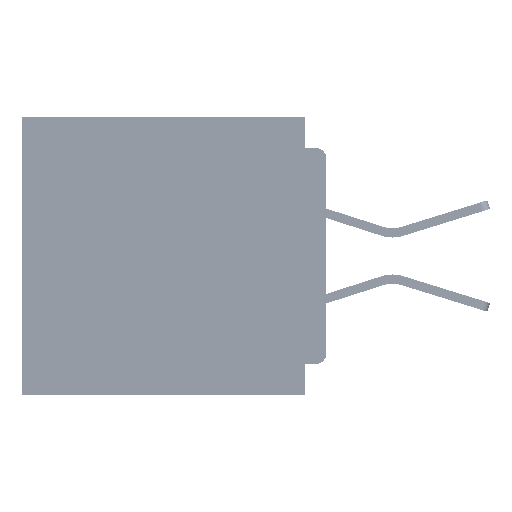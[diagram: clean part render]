
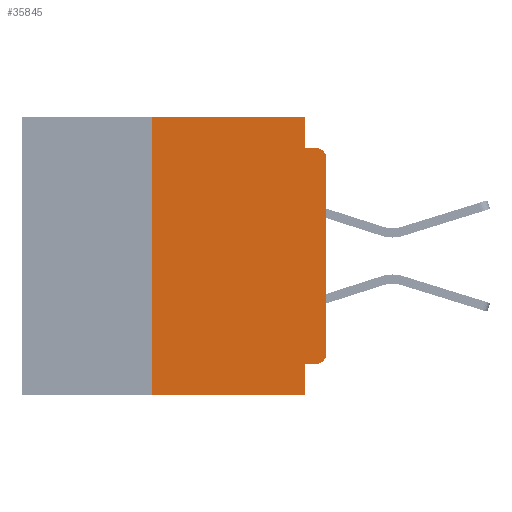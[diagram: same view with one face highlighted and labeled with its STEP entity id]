
A CAD part, left-side view. The second image highlights one B-rep face of the part: STEP entity #35845.
In plain terms, the highlighted planar face has unit normal (-1, 0, 0).
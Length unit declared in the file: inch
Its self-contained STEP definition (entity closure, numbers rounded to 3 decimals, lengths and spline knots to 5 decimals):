
#244 = CARTESIAN_POINT ( 'NONE',  ( 0., 0.015, -0.355 ) ) ;
#1551 = ORIENTED_EDGE ( 'NONE', *, *, #63702, .T. ) ;
#1789 = EDGE_CURVE ( 'NONE', #35797, #10328, #59386, .T. ) ;
#1806 = LINE ( 'NONE', #19027, #3390 ) ;
#1905 = CARTESIAN_POINT ( 'NONE',  ( 0., 0.031, 0. ) ) ;
#1924 = ORIENTED_EDGE ( 'NONE', *, *, #1789, .F. ) ;
#2128 = LINE ( 'NONE', #11401, #40152 ) ;
#2168 = CARTESIAN_POINT ( 'NONE',  ( 0., 0.015, -0.06 ) ) ;
#2187 = VECTOR ( 'NONE', #39915, 39.37008 ) ;
#2504 = CARTESIAN_POINT ( 'NONE',  ( 0., 0., -0.34 ) ) ;
#2938 = CARTESIAN_POINT ( 'NONE',  ( 0., 0.437, 0. ) ) ;
#3390 = VECTOR ( 'NONE', #53402, 39.37008 ) ;
#4965 = LINE ( 'NONE', #25827, #50999 ) ;
#5043 = VERTEX_POINT ( 'NONE', #46649 ) ;
#5642 = VERTEX_POINT ( 'NONE', #61144 ) ;
#5812 = ORIENTED_EDGE ( 'NONE', *, *, #53778, .F. ) ;
#7202 = DIRECTION ( 'NONE',  ( 0., 0., -1. ) ) ;
#8496 = CIRCLE ( 'NONE', #30777, 0.015 ) ;
#9532 = VERTEX_POINT ( 'NONE', #44308 ) ;
#10328 = VERTEX_POINT ( 'NONE', #20919 ) ;
#11029 = VECTOR ( 'NONE', #19055, 39.37008 ) ;
#11401 = CARTESIAN_POINT ( 'NONE',  ( 0., 0., -0.355 ) ) ;
#12328 = CARTESIAN_POINT ( 'NONE',  ( 0., 0.031, -0.355 ) ) ;
#16078 = EDGE_CURVE ( 'NONE', #16229, #5642, #37769, .T. ) ;
#16229 = VERTEX_POINT ( 'NONE', #36958 ) ;
#16408 = ORIENTED_EDGE ( 'NONE', *, *, #16078, .T. ) ;
#17338 = VERTEX_POINT ( 'NONE', #1905 ) ;
#17654 = AXIS2_PLACEMENT_3D ( 'NONE', #2938, #22977, #57321 ) ;
#17775 = VECTOR ( 'NONE', #53005, 39.37008 ) ;
#17961 = PLANE ( 'NONE',  #17654 ) ;
#19027 = CARTESIAN_POINT ( 'NONE',  ( 0., 0.031, 0. ) ) ;
#19055 = DIRECTION ( 'NONE',  ( 0., 0., 1. ) ) ;
#19332 = VERTEX_POINT ( 'NONE', #2504 ) ;
#19352 = LINE ( 'NONE', #23645, #17775 ) ;
#20592 = ORIENTED_EDGE ( 'NONE', *, *, #63254, .T. ) ;
#20596 = FACE_OUTER_BOUND ( 'NONE', #39555, .T. ) ;
#20919 = CARTESIAN_POINT ( 'NONE',  ( 0., 0.031, -0.4 ) ) ;
#21059 = LINE ( 'NONE', #56653, #45706 ) ;
#22080 = EDGE_CURVE ( 'NONE', #17338, #55985, #1806, .T. ) ;
#22321 = DIRECTION ( 'NONE',  ( 0., -1., 0. ) ) ;
#22477 = DIRECTION ( 'NONE',  ( -1., 0., 0. ) ) ;
#22977 = DIRECTION ( 'NONE',  ( 1., 0., 0. ) ) ;
#23645 = CARTESIAN_POINT ( 'NONE',  ( 0., 0., 0. ) ) ;
#23771 = EDGE_CURVE ( 'NONE', #9532, #10328, #21059, .T. ) ;
#24034 = ORIENTED_EDGE ( 'NONE', *, *, #32883, .F. ) ;
#24273 = LINE ( 'NONE', #38946, #11029 ) ;
#25256 = EDGE_CURVE ( 'NONE', #9532, #5043, #24273, .T. ) ;
#25827 = CARTESIAN_POINT ( 'NONE',  ( 0., 0., -0.045 ) ) ;
#27079 = ORIENTED_EDGE ( 'NONE', *, *, #25256, .F. ) ;
#27322 = EDGE_CURVE ( 'NONE', #38421, #35797, #2128, .T. ) ;
#27824 = AXIS2_PLACEMENT_3D ( 'NONE', #2168, #36883, #7202 ) ;
#30777 = AXIS2_PLACEMENT_3D ( 'NONE', #51876, #22477, #56806 ) ;
#32883 = EDGE_CURVE ( 'NONE', #55985, #5642, #4965, .T. ) ;
#35797 = VERTEX_POINT ( 'NONE', #12328 ) ;
#35845 = ADVANCED_FACE ( 'NONE', ( #20596 ), #17961, .F. ) ;
#36883 = DIRECTION ( 'NONE',  ( -1., 0., 0. ) ) ;
#36958 = CARTESIAN_POINT ( 'NONE',  ( 0., 0., -0.06 ) ) ;
#37769 = CIRCLE ( 'NONE', #27824, 0.015 ) ;
#38209 = CARTESIAN_POINT ( 'NONE',  ( 0., 0.031, -0.4 ) ) ;
#38421 = VERTEX_POINT ( 'NONE', #244 ) ;
#38946 = CARTESIAN_POINT ( 'NONE',  ( 0., 0.25, -0.4 ) ) ;
#39555 = EDGE_LOOP ( 'NONE', ( #20592, #16408, #24034, #61235, #5812, #27079, #40050, #1924, #41429, #1551 ) ) ;
#39915 = DIRECTION ( 'NONE',  ( 0., -1., 0. ) ) ;
#40050 = ORIENTED_EDGE ( 'NONE', *, *, #23771, .T. ) ;
#40152 = VECTOR ( 'NONE', #41055, 39.37008 ) ;
#41055 = DIRECTION ( 'NONE',  ( 0., 1., 0. ) ) ;
#41429 = ORIENTED_EDGE ( 'NONE', *, *, #27322, .F. ) ;
#41767 = LINE ( 'NONE', #54437, #2187 ) ;
#44308 = CARTESIAN_POINT ( 'NONE',  ( 0., 0.25, -0.4 ) ) ;
#45706 = VECTOR ( 'NONE', #22321, 39.37008 ) ;
#46376 = VECTOR ( 'NONE', #62775, 39.37008 ) ;
#46649 = CARTESIAN_POINT ( 'NONE',  ( 0., 0.25, 0. ) ) ;
#50999 = VECTOR ( 'NONE', #60184, 39.37008 ) ;
#51876 = CARTESIAN_POINT ( 'NONE',  ( 0., 0.015, -0.34 ) ) ;
#52861 = CARTESIAN_POINT ( 'NONE',  ( 0., 0.031, -0.045 ) ) ;
#53005 = DIRECTION ( 'NONE',  ( 0., 0., 1. ) ) ;
#53402 = DIRECTION ( 'NONE',  ( 0., 0., -1. ) ) ;
#53778 = EDGE_CURVE ( 'NONE', #5043, #17338, #41767, .T. ) ;
#54437 = CARTESIAN_POINT ( 'NONE',  ( 0., 0.437, 0. ) ) ;
#55985 = VERTEX_POINT ( 'NONE', #52861 ) ;
#56653 = CARTESIAN_POINT ( 'NONE',  ( 0., 0.437, -0.4 ) ) ;
#56806 = DIRECTION ( 'NONE',  ( 0., 0., -1. ) ) ;
#57321 = DIRECTION ( 'NONE',  ( 0., 0., -1. ) ) ;
#59386 = LINE ( 'NONE', #38209, #46376 ) ;
#60184 = DIRECTION ( 'NONE',  ( 0., -1., 0. ) ) ;
#61144 = CARTESIAN_POINT ( 'NONE',  ( 0., 0.015, -0.045 ) ) ;
#61235 = ORIENTED_EDGE ( 'NONE', *, *, #22080, .F. ) ;
#62775 = DIRECTION ( 'NONE',  ( 0., 0., -1. ) ) ;
#63254 = EDGE_CURVE ( 'NONE', #19332, #16229, #19352, .T. ) ;
#63702 = EDGE_CURVE ( 'NONE', #38421, #19332, #8496, .T. ) ;
